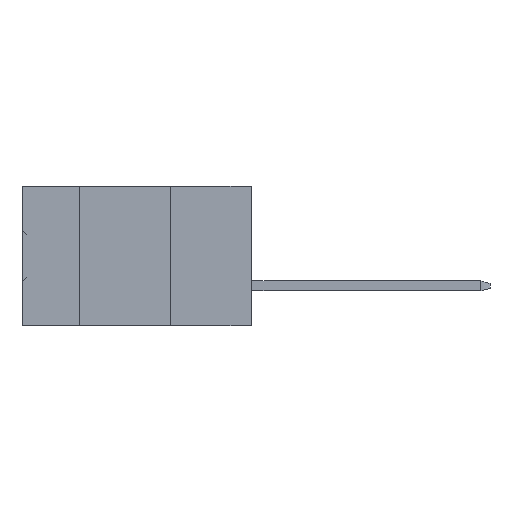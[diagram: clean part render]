
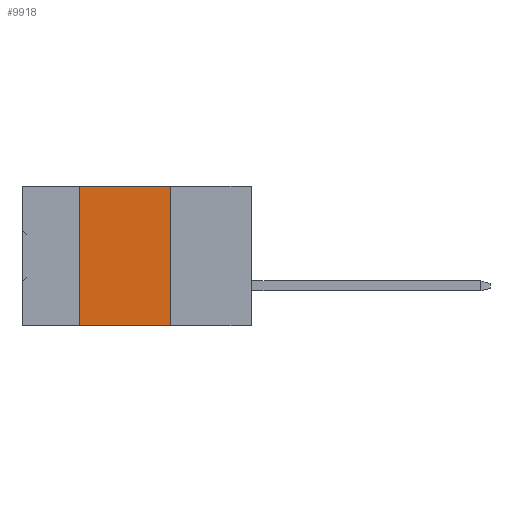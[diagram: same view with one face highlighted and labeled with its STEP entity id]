
A CAD part, left-side view. The second image highlights one B-rep face of the part: STEP entity #9918.
In plain terms, the highlighted planar face has unit normal (-1, 0, 0).
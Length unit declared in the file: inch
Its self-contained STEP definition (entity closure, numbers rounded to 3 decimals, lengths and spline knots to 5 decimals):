
#820 = CARTESIAN_POINT ( 'NONE',  ( 0., 0.72, 0. ) ) ;
#3188 = PLANE ( 'NONE',  #27537 ) ;
#6252 = LINE ( 'NONE', #18561, #30865 ) ;
#6338 = VECTOR ( 'NONE', #26093, 39.37008 ) ;
#8081 = CARTESIAN_POINT ( 'NONE',  ( 0., 0.72, 0. ) ) ;
#8228 = DIRECTION ( 'NONE',  ( 0., -1., 0. ) ) ;
#8757 = VERTEX_POINT ( 'NONE', #30854 ) ;
#8778 = DIRECTION ( 'NONE',  ( 0., 0., 1. ) ) ;
#9517 = VECTOR ( 'NONE', #8228, 39.37008 ) ;
#9918 = ADVANCED_FACE ( 'NONE', ( #17993 ), #3188, .F. ) ;
#10265 = DIRECTION ( 'NONE',  ( 1., 0., 0. ) ) ;
#10557 = VERTEX_POINT ( 'NONE', #21231 ) ;
#11350 = VECTOR ( 'NONE', #22500, 39.37008 ) ;
#11879 = CARTESIAN_POINT ( 'NONE',  ( 0., 0.254, -0.437 ) ) ;
#12919 = CARTESIAN_POINT ( 'NONE',  ( 0., 0.254, -0.437 ) ) ;
#13292 = EDGE_LOOP ( 'NONE', ( #19184, #23525, #16012, #17070 ) ) ;
#15461 = DIRECTION ( 'NONE',  ( 0., 0., -1. ) ) ;
#15931 = CARTESIAN_POINT ( 'NONE',  ( 0., 0.54, 0. ) ) ;
#16012 = ORIENTED_EDGE ( 'NONE', *, *, #20907, .F. ) ;
#17070 = ORIENTED_EDGE ( 'NONE', *, *, #26557, .T. ) ;
#17544 = LINE ( 'NONE', #8081, #9517 ) ;
#17993 = FACE_OUTER_BOUND ( 'NONE', #13292, .T. ) ;
#18561 = CARTESIAN_POINT ( 'NONE',  ( 0., 0.54, -0.437 ) ) ;
#19184 = ORIENTED_EDGE ( 'NONE', *, *, #26261, .F. ) ;
#20089 = VERTEX_POINT ( 'NONE', #11879 ) ;
#20907 = EDGE_CURVE ( 'NONE', #10557, #25364, #6252, .T. ) ;
#21231 = CARTESIAN_POINT ( 'NONE',  ( 0., 0.54, -0.437 ) ) ;
#22500 = DIRECTION ( 'NONE',  ( 0., 0., -1. ) ) ;
#23525 = ORIENTED_EDGE ( 'NONE', *, *, #31079, .F. ) ;
#25364 = VERTEX_POINT ( 'NONE', #15931 ) ;
#26093 = DIRECTION ( 'NONE',  ( 0., -1., 0. ) ) ;
#26261 = EDGE_CURVE ( 'NONE', #8757, #20089, #29555, .T. ) ;
#26557 = EDGE_CURVE ( 'NONE', #10557, #20089, #30964, .T. ) ;
#27537 = AXIS2_PLACEMENT_3D ( 'NONE', #820, #10265, #15461 ) ;
#29055 = CARTESIAN_POINT ( 'NONE',  ( 0., 0.72, -0.437 ) ) ;
#29555 = LINE ( 'NONE', #12919, #11350 ) ;
#30854 = CARTESIAN_POINT ( 'NONE',  ( 0., 0.254, 0. ) ) ;
#30865 = VECTOR ( 'NONE', #8778, 39.37008 ) ;
#30964 = LINE ( 'NONE', #29055, #6338 ) ;
#31079 = EDGE_CURVE ( 'NONE', #25364, #8757, #17544, .T. ) ;
